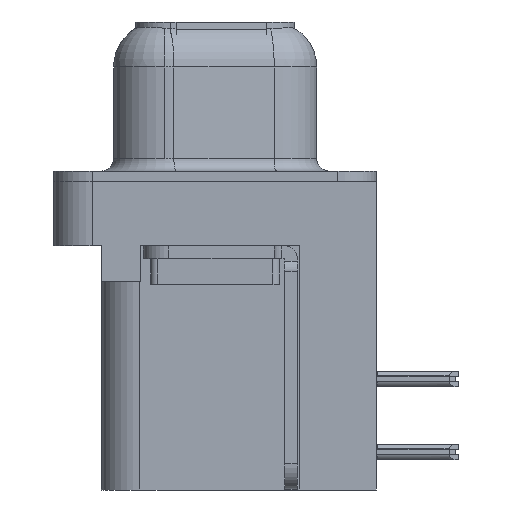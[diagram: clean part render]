
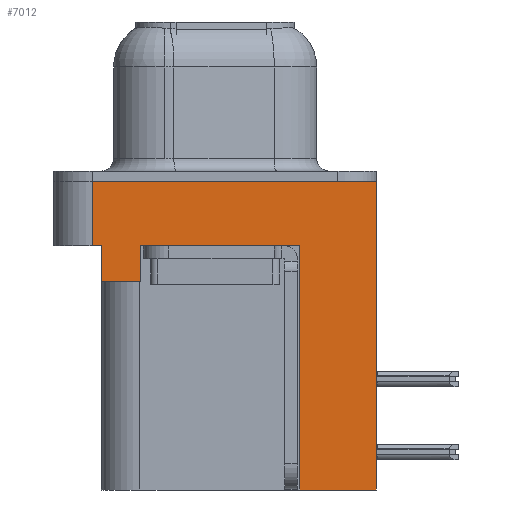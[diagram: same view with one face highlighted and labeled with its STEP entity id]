
A CAD part, left-side view. The second image highlights one B-rep face of the part: STEP entity #7012.
In plain terms, the highlighted planar face has unit normal (-1, 0, 0).
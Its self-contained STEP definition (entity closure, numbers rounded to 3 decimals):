
#274 = ORIENTED_EDGE ( 'NONE', *, *, #32939, .T. ) ;
#572 = FACE_OUTER_BOUND ( 'NONE', #18692, .T. ) ;
#1834 = CARTESIAN_POINT ( 'NONE',  ( -2.91, 4.425, -3.9 ) ) ;
#2154 = DIRECTION ( 'NONE',  ( 0., 0., 1. ) ) ;
#2326 = AXIS2_PLACEMENT_3D ( 'NONE', #24471, #24240, #2154 ) ;
#2507 = CARTESIAN_POINT ( 'NONE',  ( -2.91, 4.775, -2.5 ) ) ;
#2584 = LINE ( 'NONE', #34049, #16841 ) ;
#2636 = CARTESIAN_POINT ( 'NONE',  ( -2.91, 4.775, 0. ) ) ;
#2792 = VECTOR ( 'NONE', #8436, 1000. ) ;
#3881 = CARTESIAN_POINT ( 'NONE',  ( -2.91, 2.895, -3.9 ) ) ;
#4143 = EDGE_CURVE ( 'NONE', #29192, #28928, #2584, .T. ) ;
#4407 = CARTESIAN_POINT ( 'NONE',  ( -2.91, -6.275, -2.5 ) ) ;
#4566 = CARTESIAN_POINT ( 'NONE',  ( -2.91, -3.295, -12. ) ) ;
#5232 = EDGE_CURVE ( 'NONE', #19823, #15069, #13288, .T. ) ;
#5301 = EDGE_CURVE ( 'NONE', #29322, #29192, #6369, .T. ) ;
#5676 = VERTEX_POINT ( 'NONE', #7846 ) ;
#6083 = CARTESIAN_POINT ( 'NONE',  ( -2.91, -3.295, -2.5 ) ) ;
#6369 = LINE ( 'NONE', #2507, #15936 ) ;
#6771 = ORIENTED_EDGE ( 'NONE', *, *, #13193, .T. ) ;
#7012 = ADVANCED_FACE ( 'NONE', ( #572 ), #9735, .T. ) ;
#7374 = DIRECTION ( 'NONE',  ( 0., 1., 0. ) ) ;
#7846 = CARTESIAN_POINT ( 'NONE',  ( -2.91, -6.275, -12. ) ) ;
#7960 = ORIENTED_EDGE ( 'NONE', *, *, #13763, .T. ) ;
#8436 = DIRECTION ( 'NONE',  ( 0., 0., 1. ) ) ;
#8585 = VECTOR ( 'NONE', #12060, 1000. ) ;
#8671 = EDGE_CURVE ( 'NONE', #10638, #35832, #30289, .T. ) ;
#8897 = ORIENTED_EDGE ( 'NONE', *, *, #5301, .F. ) ;
#9735 = PLANE ( 'NONE',  #2326 ) ;
#10628 = EDGE_CURVE ( 'NONE', #5676, #15024, #15752, .T. ) ;
#10638 = VERTEX_POINT ( 'NONE', #28076 ) ;
#11585 = DIRECTION ( 'NONE',  ( 0., -1., 0. ) ) ;
#12060 = DIRECTION ( 'NONE',  ( 0., 0., 1. ) ) ;
#12476 = VECTOR ( 'NONE', #16343, 1000. ) ;
#13193 = EDGE_CURVE ( 'NONE', #30699, #10638, #27242, .T. ) ;
#13288 = LINE ( 'NONE', #29895, #31537 ) ;
#13531 = VECTOR ( 'NONE', #28494, 1000. ) ;
#13763 = EDGE_CURVE ( 'NONE', #5676, #28928, #23157, .T. ) ;
#13913 = CARTESIAN_POINT ( 'NONE',  ( -2.91, -6.275, -2.5 ) ) ;
#14109 = ORIENTED_EDGE ( 'NONE', *, *, #5232, .F. ) ;
#14471 = ORIENTED_EDGE ( 'NONE', *, *, #4143, .F. ) ;
#15024 = VERTEX_POINT ( 'NONE', #24789 ) ;
#15069 = VERTEX_POINT ( 'NONE', #27995 ) ;
#15248 = ORIENTED_EDGE ( 'NONE', *, *, #10628, .F. ) ;
#15752 = LINE ( 'NONE', #4566, #13531 ) ;
#15783 = EDGE_CURVE ( 'NONE', #15024, #35832, #31186, .T. ) ;
#15936 = VECTOR ( 'NONE', #27446, 1000. ) ;
#16343 = DIRECTION ( 'NONE',  ( 0., 0., 1. ) ) ;
#16841 = VECTOR ( 'NONE', #11585, 1000. ) ;
#17922 = ORIENTED_EDGE ( 'NONE', *, *, #15783, .F. ) ;
#18692 = EDGE_LOOP ( 'NONE', ( #14471, #8897, #274, #14109, #24104, #6771, #20108, #17922, #15248, #7960 ) ) ;
#19036 = CARTESIAN_POINT ( 'NONE',  ( -2.91, -6.275, -2.5 ) ) ;
#19056 = CARTESIAN_POINT ( 'NONE',  ( -2.91, -6.275, 0. ) ) ;
#19142 = DIRECTION ( 'NONE',  ( 0., -1., 0. ) ) ;
#19823 = VERTEX_POINT ( 'NONE', #28662 ) ;
#20028 = VECTOR ( 'NONE', #7374, 1000. ) ;
#20108 = ORIENTED_EDGE ( 'NONE', *, *, #8671, .T. ) ;
#20262 = LINE ( 'NONE', #4407, #31124 ) ;
#21530 = CARTESIAN_POINT ( 'NONE',  ( -2.91, -3.295, -12. ) ) ;
#23157 = LINE ( 'NONE', #13913, #2792 ) ;
#24104 = ORIENTED_EDGE ( 'NONE', *, *, #32070, .F. ) ;
#24240 = DIRECTION ( 'NONE',  ( -1., 0., 0. ) ) ;
#24355 = CARTESIAN_POINT ( 'NONE',  ( -2.91, 2.895, -3.9 ) ) ;
#24471 = CARTESIAN_POINT ( 'NONE',  ( -2.91, -6.275, -2.5 ) ) ;
#24789 = CARTESIAN_POINT ( 'NONE',  ( -2.91, -3.295, -12. ) ) ;
#26545 = LINE ( 'NONE', #1834, #20028 ) ;
#27242 = LINE ( 'NONE', #24355, #12476 ) ;
#27252 = VECTOR ( 'NONE', #19142, 1000. ) ;
#27323 = DIRECTION ( 'NONE',  ( 0., 0., 1. ) ) ;
#27446 = DIRECTION ( 'NONE',  ( 0., 0., 1. ) ) ;
#27995 = CARTESIAN_POINT ( 'NONE',  ( -2.91, 4.425, -2.5 ) ) ;
#28076 = CARTESIAN_POINT ( 'NONE',  ( -2.91, 2.895, -2.5 ) ) ;
#28296 = CARTESIAN_POINT ( 'NONE',  ( -2.91, 4.775, -2.5 ) ) ;
#28494 = DIRECTION ( 'NONE',  ( 0., 1., 0. ) ) ;
#28662 = CARTESIAN_POINT ( 'NONE',  ( -2.91, 4.425, -3.9 ) ) ;
#28928 = VERTEX_POINT ( 'NONE', #19056 ) ;
#29192 = VERTEX_POINT ( 'NONE', #2636 ) ;
#29322 = VERTEX_POINT ( 'NONE', #28296 ) ;
#29355 = DIRECTION ( 'NONE',  ( 0., -1., 0. ) ) ;
#29895 = CARTESIAN_POINT ( 'NONE',  ( -2.91, 4.425, -3.9 ) ) ;
#30289 = LINE ( 'NONE', #19036, #27252 ) ;
#30699 = VERTEX_POINT ( 'NONE', #3881 ) ;
#31124 = VECTOR ( 'NONE', #29355, 1000. ) ;
#31186 = LINE ( 'NONE', #21530, #8585 ) ;
#31537 = VECTOR ( 'NONE', #27323, 1000. ) ;
#32070 = EDGE_CURVE ( 'NONE', #30699, #19823, #26545, .T. ) ;
#32939 = EDGE_CURVE ( 'NONE', #29322, #15069, #20262, .T. ) ;
#34049 = CARTESIAN_POINT ( 'NONE',  ( -2.91, -6.275, 0. ) ) ;
#35832 = VERTEX_POINT ( 'NONE', #6083 ) ;
